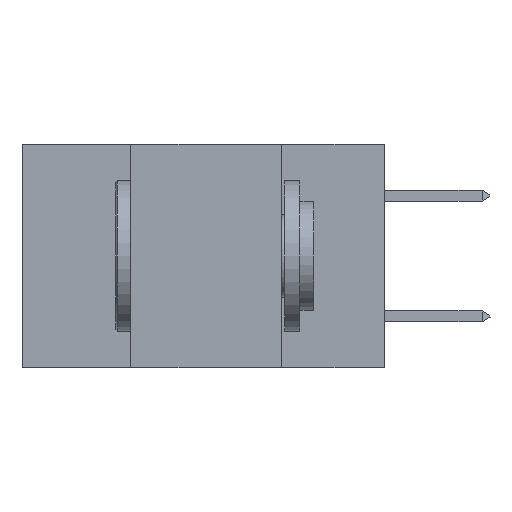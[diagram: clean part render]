
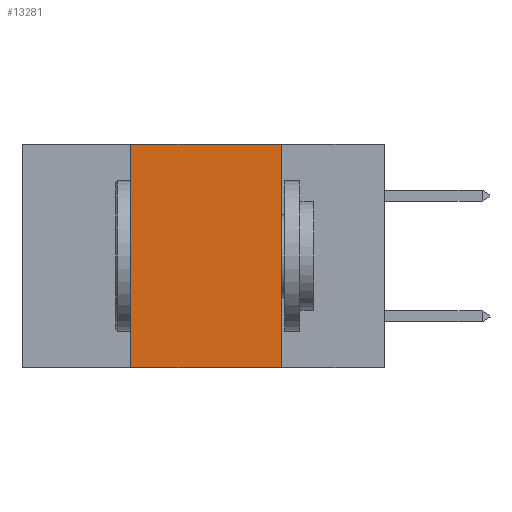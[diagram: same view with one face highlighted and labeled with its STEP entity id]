
A CAD part, left-side view. The second image highlights one B-rep face of the part: STEP entity #13281.
In plain terms, the highlighted planar face has unit normal (-1, 0, 0).
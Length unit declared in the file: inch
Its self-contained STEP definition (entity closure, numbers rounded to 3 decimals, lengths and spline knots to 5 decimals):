
#509 = ORIENTED_EDGE ( 'NONE', *, *, #2401, .F. ) ;
#1629 = CARTESIAN_POINT ( 'NONE',  ( 0., 0.17, 0. ) ) ;
#1734 = VECTOR ( 'NONE', #30683, 39.37008 ) ;
#2401 = EDGE_CURVE ( 'NONE', #15512, #16803, #10733, .T. ) ;
#2549 = VERTEX_POINT ( 'NONE', #11557 ) ;
#2738 = FACE_OUTER_BOUND ( 'NONE', #13061, .T. ) ;
#4569 = ORIENTED_EDGE ( 'NONE', *, *, #16690, .T. ) ;
#4898 = VECTOR ( 'NONE', #34493, 39.37008 ) ;
#6565 = CARTESIAN_POINT ( 'NONE',  ( 0., 0.6, 0. ) ) ;
#6825 = CARTESIAN_POINT ( 'NONE',  ( 0., 0.42, 0. ) ) ;
#8515 = AXIS2_PLACEMENT_3D ( 'NONE', #26317, #17407, #20243 ) ;
#9068 = EDGE_CURVE ( 'NONE', #17536, #15512, #28699, .T. ) ;
#10733 = LINE ( 'NONE', #1629, #23972 ) ;
#11557 = CARTESIAN_POINT ( 'NONE',  ( 0., 0.42, -0.37 ) ) ;
#11599 = CARTESIAN_POINT ( 'NONE',  ( 0., 0.17, -0.37 ) ) ;
#13061 = EDGE_LOOP ( 'NONE', ( #509, #19406, #28062, #4569 ) ) ;
#13281 = ADVANCED_FACE ( 'NONE', ( #2738 ), #14552, .F. ) ;
#14552 = PLANE ( 'NONE',  #8515 ) ;
#15512 = VERTEX_POINT ( 'NONE', #34586 ) ;
#16690 = EDGE_CURVE ( 'NONE', #2549, #16803, #29514, .T. ) ;
#16794 = VECTOR ( 'NONE', #20922, 39.37008 ) ;
#16803 = VERTEX_POINT ( 'NONE', #11599 ) ;
#17407 = DIRECTION ( 'NONE',  ( 1., 0., 0. ) ) ;
#17536 = VERTEX_POINT ( 'NONE', #24667 ) ;
#18710 = DIRECTION ( 'NONE',  ( 0., 0., -1. ) ) ;
#19406 = ORIENTED_EDGE ( 'NONE', *, *, #9068, .F. ) ;
#20243 = DIRECTION ( 'NONE',  ( 0., 0., -1. ) ) ;
#20922 = DIRECTION ( 'NONE',  ( 0., 0., 1. ) ) ;
#23972 = VECTOR ( 'NONE', #18710, 39.37008 ) ;
#24326 = LINE ( 'NONE', #6825, #16794 ) ;
#24667 = CARTESIAN_POINT ( 'NONE',  ( 0., 0.42, 0. ) ) ;
#26317 = CARTESIAN_POINT ( 'NONE',  ( 0., 0.6, 0. ) ) ;
#28062 = ORIENTED_EDGE ( 'NONE', *, *, #34657, .F. ) ;
#28699 = LINE ( 'NONE', #6565, #4898 ) ;
#29514 = LINE ( 'NONE', #33512, #1734 ) ;
#30683 = DIRECTION ( 'NONE',  ( 0., -1., 0. ) ) ;
#33512 = CARTESIAN_POINT ( 'NONE',  ( 0., 0.6, -0.37 ) ) ;
#34493 = DIRECTION ( 'NONE',  ( 0., -1., 0. ) ) ;
#34586 = CARTESIAN_POINT ( 'NONE',  ( 0., 0.17, 0. ) ) ;
#34657 = EDGE_CURVE ( 'NONE', #2549, #17536, #24326, .T. ) ;
